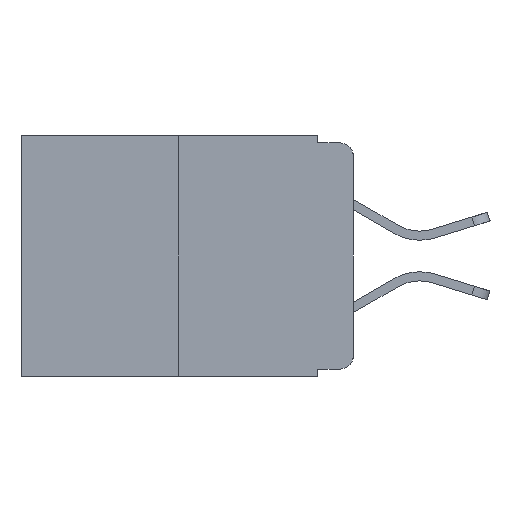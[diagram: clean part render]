
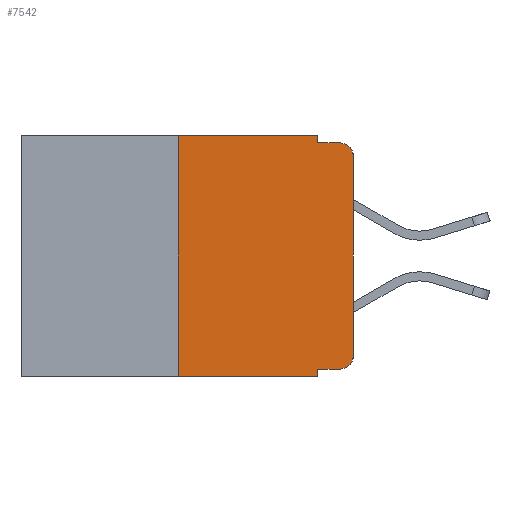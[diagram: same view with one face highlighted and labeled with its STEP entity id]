
A CAD part, left-side view. The second image highlights one B-rep face of the part: STEP entity #7542.
In plain terms, the highlighted planar face has unit normal (-1, 0, 0).
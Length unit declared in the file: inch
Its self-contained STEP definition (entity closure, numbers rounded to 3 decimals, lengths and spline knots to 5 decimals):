
#199 = ORIENTED_EDGE ( 'NONE', *, *, #10043, .F. ) ;
#371 = AXIS2_PLACEMENT_3D ( 'NONE', #6618, #1344, #7424 ) ;
#440 = EDGE_CURVE ( 'NONE', #5093, #2041, #10415, .T. ) ;
#480 = ORIENTED_EDGE ( 'NONE', *, *, #6633, .F. ) ;
#578 = EDGE_CURVE ( 'NONE', #3449, #7066, #7303, .T. ) ;
#678 = VECTOR ( 'NONE', #687, 39.37008 ) ;
#686 = CARTESIAN_POINT ( 'NONE',  ( 0., 0.473, 0. ) ) ;
#687 = DIRECTION ( 'NONE',  ( 0., -1., 0. ) ) ;
#829 = DIRECTION ( 'NONE',  ( 0., 0., -1. ) ) ;
#871 = CARTESIAN_POINT ( 'NONE',  ( 0., 0.051, 0. ) ) ;
#1042 = LINE ( 'NONE', #4470, #6947 ) ;
#1190 = CARTESIAN_POINT ( 'NONE',  ( 0., 0.25, 0. ) ) ;
#1344 = DIRECTION ( 'NONE',  ( 1., 0., 0. ) ) ;
#1352 = ORIENTED_EDGE ( 'NONE', *, *, #7216, .F. ) ;
#1645 = CARTESIAN_POINT ( 'NONE',  ( 0., 0., 0. ) ) ;
#1922 = EDGE_CURVE ( 'NONE', #10718, #3806, #2956, .T. ) ;
#2041 = VERTEX_POINT ( 'NONE', #2907 ) ;
#2120 = VERTEX_POINT ( 'NONE', #3531 ) ;
#2267 = VERTEX_POINT ( 'NONE', #5615 ) ;
#2349 = VERTEX_POINT ( 'NONE', #2943 ) ;
#2543 = ORIENTED_EDGE ( 'NONE', *, *, #6134, .F. ) ;
#2590 = CARTESIAN_POINT ( 'NONE',  ( 0., 0.473, -0.343 ) ) ;
#2603 = DIRECTION ( 'NONE',  ( 0., 0., -1. ) ) ;
#2622 = EDGE_CURVE ( 'NONE', #2349, #3449, #5122, .T. ) ;
#2681 = CIRCLE ( 'NONE', #6895, 0.02 ) ;
#2697 = FACE_OUTER_BOUND ( 'NONE', #8072, .T. ) ;
#2907 = CARTESIAN_POINT ( 'NONE',  ( 0., 0.051, -0.343 ) ) ;
#2910 = DIRECTION ( 'NONE',  ( 0., -1., 0. ) ) ;
#2943 = CARTESIAN_POINT ( 'NONE',  ( 0., 0.051, -0.333 ) ) ;
#2956 = LINE ( 'NONE', #8087, #5274 ) ;
#3220 = CARTESIAN_POINT ( 'NONE',  ( 0., 0.051, -0.01 ) ) ;
#3248 = DIRECTION ( 'NONE',  ( -1., 0., 0. ) ) ;
#3430 = DIRECTION ( 'NONE',  ( 0., -1., 0. ) ) ;
#3449 = VERTEX_POINT ( 'NONE', #5255 ) ;
#3531 = CARTESIAN_POINT ( 'NONE',  ( 0., 0., -0.03 ) ) ;
#3591 = ORIENTED_EDGE ( 'NONE', *, *, #578, .T. ) ;
#3806 = VERTEX_POINT ( 'NONE', #5506 ) ;
#3994 = ORIENTED_EDGE ( 'NONE', *, *, #5468, .T. ) ;
#4349 = VECTOR ( 'NONE', #3430, 39.37008 ) ;
#4436 = DIRECTION ( 'NONE',  ( 0., 0., 1. ) ) ;
#4470 = CARTESIAN_POINT ( 'NONE',  ( 0., 0.051, 0. ) ) ;
#4531 = LINE ( 'NONE', #1645, #10827 ) ;
#4872 = LINE ( 'NONE', #1190, #9304 ) ;
#5072 = ORIENTED_EDGE ( 'NONE', *, *, #9838, .T. ) ;
#5093 = VERTEX_POINT ( 'NONE', #6322 ) ;
#5122 = LINE ( 'NONE', #5964, #678 ) ;
#5255 = CARTESIAN_POINT ( 'NONE',  ( 0., 0.02, -0.333 ) ) ;
#5274 = VECTOR ( 'NONE', #2910, 39.37008 ) ;
#5363 = DIRECTION ( 'NONE',  ( 0., 0., -1. ) ) ;
#5468 = EDGE_CURVE ( 'NONE', #7066, #2120, #4531, .T. ) ;
#5506 = CARTESIAN_POINT ( 'NONE',  ( 0., 0.02, -0.01 ) ) ;
#5614 = DIRECTION ( 'NONE',  ( 0., 0., 1. ) ) ;
#5615 = CARTESIAN_POINT ( 'NONE',  ( 0., 0.051, 0. ) ) ;
#5964 = CARTESIAN_POINT ( 'NONE',  ( 0., 0.051, -0.333 ) ) ;
#6134 = EDGE_CURVE ( 'NONE', #2349, #2041, #1042, .T. ) ;
#6159 = DIRECTION ( 'NONE',  ( -1., 0., 0. ) ) ;
#6171 = LINE ( 'NONE', #686, #8089 ) ;
#6322 = CARTESIAN_POINT ( 'NONE',  ( 0., 0.25, -0.343 ) ) ;
#6618 = CARTESIAN_POINT ( 'NONE',  ( 0., 0.473, 0. ) ) ;
#6633 = EDGE_CURVE ( 'NONE', #10524, #2267, #6171, .T. ) ;
#6883 = DIRECTION ( 'NONE',  ( 0., -1., 0. ) ) ;
#6895 = AXIS2_PLACEMENT_3D ( 'NONE', #10936, #6159, #829 ) ;
#6947 = VECTOR ( 'NONE', #5363, 39.37008 ) ;
#7016 = DIRECTION ( 'NONE',  ( 0., 0., -1. ) ) ;
#7066 = VERTEX_POINT ( 'NONE', #7612 ) ;
#7107 = CARTESIAN_POINT ( 'NONE',  ( 0., 0.02, -0.313 ) ) ;
#7216 = EDGE_CURVE ( 'NONE', #2267, #10718, #8443, .T. ) ;
#7303 = CIRCLE ( 'NONE', #8489, 0.02 ) ;
#7424 = DIRECTION ( 'NONE',  ( 0., 0., -1. ) ) ;
#7542 = ADVANCED_FACE ( 'NONE', ( #2697 ), #10595, .F. ) ;
#7612 = CARTESIAN_POINT ( 'NONE',  ( 0., 0., -0.313 ) ) ;
#8072 = EDGE_LOOP ( 'NONE', ( #3994, #5072, #9479, #1352, #480, #199, #8919, #2543, #8888, #3591 ) ) ;
#8087 = CARTESIAN_POINT ( 'NONE',  ( 0., 0.051, -0.01 ) ) ;
#8089 = VECTOR ( 'NONE', #6883, 39.37008 ) ;
#8443 = LINE ( 'NONE', #871, #10280 ) ;
#8489 = AXIS2_PLACEMENT_3D ( 'NONE', #7107, #3248, #2603 ) ;
#8748 = CARTESIAN_POINT ( 'NONE',  ( 0., 0.25, 0. ) ) ;
#8888 = ORIENTED_EDGE ( 'NONE', *, *, #2622, .T. ) ;
#8919 = ORIENTED_EDGE ( 'NONE', *, *, #440, .T. ) ;
#9304 = VECTOR ( 'NONE', #5614, 39.37008 ) ;
#9479 = ORIENTED_EDGE ( 'NONE', *, *, #1922, .F. ) ;
#9838 = EDGE_CURVE ( 'NONE', #2120, #3806, #2681, .T. ) ;
#10043 = EDGE_CURVE ( 'NONE', #5093, #10524, #4872, .T. ) ;
#10280 = VECTOR ( 'NONE', #7016, 39.37008 ) ;
#10415 = LINE ( 'NONE', #2590, #4349 ) ;
#10524 = VERTEX_POINT ( 'NONE', #8748 ) ;
#10595 = PLANE ( 'NONE',  #371 ) ;
#10718 = VERTEX_POINT ( 'NONE', #3220 ) ;
#10827 = VECTOR ( 'NONE', #4436, 39.37008 ) ;
#10936 = CARTESIAN_POINT ( 'NONE',  ( 0., 0.02, -0.03 ) ) ;
